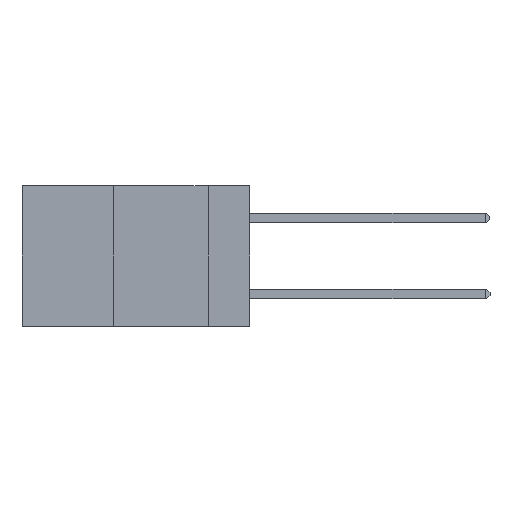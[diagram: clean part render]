
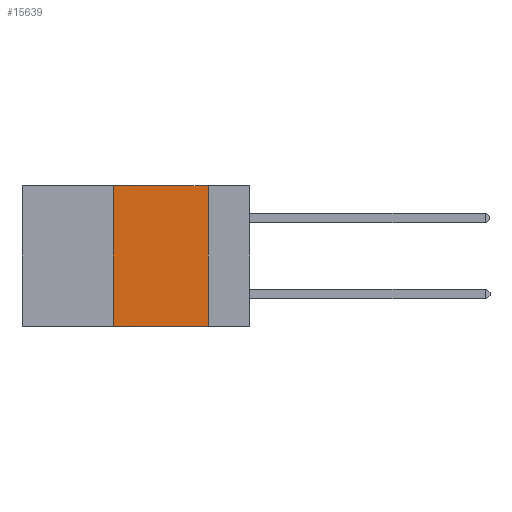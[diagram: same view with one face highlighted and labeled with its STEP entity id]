
A CAD part, left-side view. The second image highlights one B-rep face of the part: STEP entity #15639.
In plain terms, the highlighted planar face has unit normal (-1, 0, 0).
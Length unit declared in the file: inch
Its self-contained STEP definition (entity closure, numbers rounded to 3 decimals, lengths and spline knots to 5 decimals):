
#158 = DIRECTION ( 'NONE',  ( 1., 0., 0. ) ) ;
#427 = DIRECTION ( 'NONE',  ( 0., -1., 0. ) ) ;
#564 = CARTESIAN_POINT ( 'NONE',  ( 0., 0.6, 0. ) ) ;
#1888 = ORIENTED_EDGE ( 'NONE', *, *, #21740, .F. ) ;
#2046 = VECTOR ( 'NONE', #14248, 39.37008 ) ;
#2858 = VERTEX_POINT ( 'NONE', #3973 ) ;
#3830 = AXIS2_PLACEMENT_3D ( 'NONE', #21060, #158, #12546 ) ;
#3842 = DIRECTION ( 'NONE',  ( 0., 0., -1. ) ) ;
#3946 = VECTOR ( 'NONE', #427, 39.37008 ) ;
#3973 = CARTESIAN_POINT ( 'NONE',  ( 0., 0.36, 0. ) ) ;
#3986 = CARTESIAN_POINT ( 'NONE',  ( 0., 0.11, 0. ) ) ;
#4494 = LINE ( 'NONE', #21372, #3946 ) ;
#4537 = CARTESIAN_POINT ( 'NONE',  ( 0., 0.36, -0.37 ) ) ;
#6641 = ORIENTED_EDGE ( 'NONE', *, *, #20085, .F. ) ;
#6797 = LINE ( 'NONE', #12503, #2046 ) ;
#7390 = VECTOR ( 'NONE', #3842, 39.37008 ) ;
#7743 = VERTEX_POINT ( 'NONE', #3986 ) ;
#8302 = EDGE_CURVE ( 'NONE', #21978, #2858, #6797, .T. ) ;
#10079 = VERTEX_POINT ( 'NONE', #22523 ) ;
#12062 = LINE ( 'NONE', #16086, #7390 ) ;
#12503 = CARTESIAN_POINT ( 'NONE',  ( 0., 0.36, 0. ) ) ;
#12546 = DIRECTION ( 'NONE',  ( 0., 0., -1. ) ) ;
#13307 = FACE_OUTER_BOUND ( 'NONE', #17256, .T. ) ;
#14224 = PLANE ( 'NONE',  #3830 ) ;
#14248 = DIRECTION ( 'NONE',  ( 0., 0., 1. ) ) ;
#15639 = ADVANCED_FACE ( 'NONE', ( #13307 ), #14224, .F. ) ;
#15859 = VECTOR ( 'NONE', #16339, 39.37008 ) ;
#16086 = CARTESIAN_POINT ( 'NONE',  ( 0., 0.11, 0. ) ) ;
#16339 = DIRECTION ( 'NONE',  ( 0., -1., 0. ) ) ;
#16961 = ORIENTED_EDGE ( 'NONE', *, *, #17599, .T. ) ;
#17256 = EDGE_LOOP ( 'NONE', ( #1888, #6641, #21003, #16961 ) ) ;
#17599 = EDGE_CURVE ( 'NONE', #21978, #10079, #4494, .T. ) ;
#19374 = LINE ( 'NONE', #564, #15859 ) ;
#20085 = EDGE_CURVE ( 'NONE', #2858, #7743, #19374, .T. ) ;
#21003 = ORIENTED_EDGE ( 'NONE', *, *, #8302, .F. ) ;
#21060 = CARTESIAN_POINT ( 'NONE',  ( 0., 0.6, 0. ) ) ;
#21372 = CARTESIAN_POINT ( 'NONE',  ( 0., 0.6, -0.37 ) ) ;
#21740 = EDGE_CURVE ( 'NONE', #7743, #10079, #12062, .T. ) ;
#21978 = VERTEX_POINT ( 'NONE', #4537 ) ;
#22523 = CARTESIAN_POINT ( 'NONE',  ( 0., 0.11, -0.37 ) ) ;
